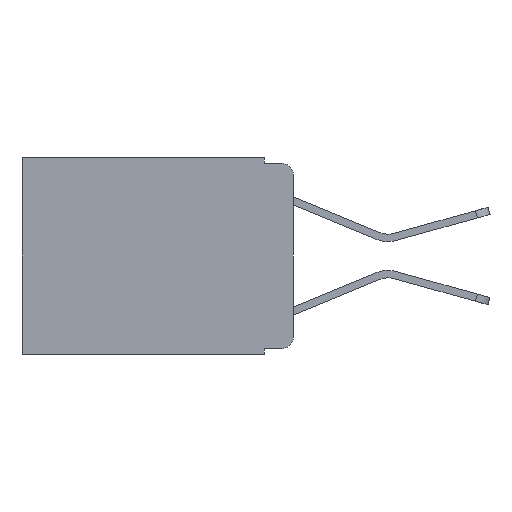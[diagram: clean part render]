
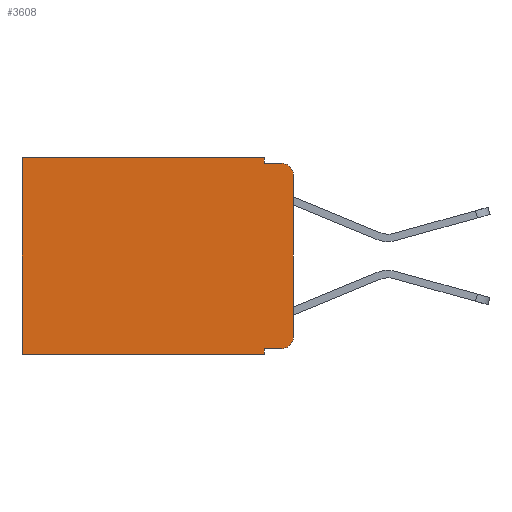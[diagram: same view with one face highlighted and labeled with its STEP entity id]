
A CAD part, left-side view. The second image highlights one B-rep face of the part: STEP entity #3608.
In plain terms, the highlighted planar face has unit normal (-1, 0, 0).
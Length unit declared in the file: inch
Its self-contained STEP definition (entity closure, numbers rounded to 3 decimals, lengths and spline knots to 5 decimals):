
#330 = VERTEX_POINT ( 'NONE', #3172 ) ;
#378 = ORIENTED_EDGE ( 'NONE', *, *, #8290, .F. ) ;
#444 = DIRECTION ( 'NONE',  ( 0., 0., -1. ) ) ;
#503 = CARTESIAN_POINT ( 'NONE',  ( 0.298, 0.051, -0.343 ) ) ;
#592 = CARTESIAN_POINT ( 'NONE',  ( 0.298, 0.02, -0.333 ) ) ;
#918 = CARTESIAN_POINT ( 'NONE',  ( 0.298, 0.051, 0. ) ) ;
#926 = VERTEX_POINT ( 'NONE', #20212 ) ;
#1026 = EDGE_CURVE ( 'NONE', #15799, #330, #22516, .T. ) ;
#1278 = LINE ( 'NONE', #4128, #19422 ) ;
#1350 = AXIS2_PLACEMENT_3D ( 'NONE', #12746, #19633, #444 ) ;
#1953 = VERTEX_POINT ( 'NONE', #12232 ) ;
#1965 = EDGE_CURVE ( 'NONE', #20426, #7676, #14026, .T. ) ;
#2195 = VECTOR ( 'NONE', #8801, 39.37008 ) ;
#2557 = VERTEX_POINT ( 'NONE', #918 ) ;
#2786 = LINE ( 'NONE', #15776, #2195 ) ;
#3076 = DIRECTION ( 'NONE',  ( 0., 0., -1. ) ) ;
#3172 = CARTESIAN_POINT ( 'NONE',  ( 0.298, 0.02, -0.01 ) ) ;
#3275 = VERTEX_POINT ( 'NONE', #503 ) ;
#3299 = ORIENTED_EDGE ( 'NONE', *, *, #6806, .T. ) ;
#3582 = DIRECTION ( 'NONE',  ( 0., 1., 0. ) ) ;
#3608 = ADVANCED_FACE ( 'NONE', ( #9942 ), #6311, .F. ) ;
#3767 = LINE ( 'NONE', #5191, #7946 ) ;
#4128 = CARTESIAN_POINT ( 'NONE',  ( 0.298, 0., 0. ) ) ;
#4423 = EDGE_CURVE ( 'NONE', #20426, #3275, #3767, .T. ) ;
#4692 = CARTESIAN_POINT ( 'NONE',  ( 0.298, 0., -0.343 ) ) ;
#5191 = CARTESIAN_POINT ( 'NONE',  ( 0.298, 0.051, 0. ) ) ;
#5262 = DIRECTION ( 'NONE',  ( -1., 0., 0. ) ) ;
#5292 = ORIENTED_EDGE ( 'NONE', *, *, #16869, .F. ) ;
#5762 = CARTESIAN_POINT ( 'NONE',  ( 0.298, 0.051, -0.333 ) ) ;
#5862 = ORIENTED_EDGE ( 'NONE', *, *, #11166, .T. ) ;
#5957 = DIRECTION ( 'NONE',  ( 0., 0., -1. ) ) ;
#6195 = VECTOR ( 'NONE', #11718, 39.37008 ) ;
#6311 = PLANE ( 'NONE',  #1350 ) ;
#6524 = DIRECTION ( 'NONE',  ( 0., 0., -1. ) ) ;
#6772 = LINE ( 'NONE', #22443, #20555 ) ;
#6806 = EDGE_CURVE ( 'NONE', #7155, #926, #21037, .T. ) ;
#7155 = VERTEX_POINT ( 'NONE', #19468 ) ;
#7283 = VECTOR ( 'NONE', #22437, 39.37008 ) ;
#7502 = ORIENTED_EDGE ( 'NONE', *, *, #1026, .T. ) ;
#7676 = VERTEX_POINT ( 'NONE', #592 ) ;
#7946 = VECTOR ( 'NONE', #6524, 39.37008 ) ;
#8290 = EDGE_CURVE ( 'NONE', #15799, #1953, #1278, .T. ) ;
#8801 = DIRECTION ( 'NONE',  ( 0., 0., -1. ) ) ;
#9430 = VECTOR ( 'NONE', #16887, 39.37008 ) ;
#9852 = VERTEX_POINT ( 'NONE', #20688 ) ;
#9942 = FACE_OUTER_BOUND ( 'NONE', #10870, .T. ) ;
#10552 = ORIENTED_EDGE ( 'NONE', *, *, #4423, .F. ) ;
#10700 = AXIS2_PLACEMENT_3D ( 'NONE', #15721, #5262, #17434 ) ;
#10870 = EDGE_LOOP ( 'NONE', ( #378, #7502, #17818, #5292, #5862, #3299, #17269, #10552, #11100, #19688 ) ) ;
#11100 = ORIENTED_EDGE ( 'NONE', *, *, #1965, .T. ) ;
#11166 = EDGE_CURVE ( 'NONE', #2557, #7155, #17694, .T. ) ;
#11718 = DIRECTION ( 'NONE',  ( 0., 1., 0. ) ) ;
#11940 = LINE ( 'NONE', #4692, #6195 ) ;
#12232 = CARTESIAN_POINT ( 'NONE',  ( 0.298, 0., -0.313 ) ) ;
#12289 = DIRECTION ( 'NONE',  ( 0., -1., 0. ) ) ;
#12746 = CARTESIAN_POINT ( 'NONE',  ( 0.298, 0., 0. ) ) ;
#13658 = DIRECTION ( 'NONE',  ( -1., 0., 0. ) ) ;
#14026 = LINE ( 'NONE', #19679, #9430 ) ;
#14209 = CARTESIAN_POINT ( 'NONE',  ( 0.298, 0., 0. ) ) ;
#15721 = CARTESIAN_POINT ( 'NONE',  ( 0.298, 0.02, -0.313 ) ) ;
#15776 = CARTESIAN_POINT ( 'NONE',  ( 0.298, 0.051, 0. ) ) ;
#15799 = VERTEX_POINT ( 'NONE', #22326 ) ;
#16662 = EDGE_CURVE ( 'NONE', #3275, #926, #11940, .T. ) ;
#16869 = EDGE_CURVE ( 'NONE', #2557, #9852, #2786, .T. ) ;
#16887 = DIRECTION ( 'NONE',  ( 0., -1., 0. ) ) ;
#17269 = ORIENTED_EDGE ( 'NONE', *, *, #16662, .F. ) ;
#17434 = DIRECTION ( 'NONE',  ( 0., 0., -1. ) ) ;
#17694 = LINE ( 'NONE', #14209, #18224 ) ;
#17818 = ORIENTED_EDGE ( 'NONE', *, *, #22482, .F. ) ;
#18224 = VECTOR ( 'NONE', #3582, 39.37008 ) ;
#18571 = CARTESIAN_POINT ( 'NONE',  ( 0.298, 0.02, -0.03 ) ) ;
#18747 = CIRCLE ( 'NONE', #10700, 0.02 ) ;
#19422 = VECTOR ( 'NONE', #5957, 39.37008 ) ;
#19468 = CARTESIAN_POINT ( 'NONE',  ( 0.298, 0.473, 0. ) ) ;
#19633 = DIRECTION ( 'NONE',  ( 1., 0., 0. ) ) ;
#19679 = CARTESIAN_POINT ( 'NONE',  ( 0.298, 0.051, -0.333 ) ) ;
#19688 = ORIENTED_EDGE ( 'NONE', *, *, #20872, .T. ) ;
#20212 = CARTESIAN_POINT ( 'NONE',  ( 0.298, 0.473, -0.343 ) ) ;
#20426 = VERTEX_POINT ( 'NONE', #5762 ) ;
#20529 = AXIS2_PLACEMENT_3D ( 'NONE', #18571, #13658, #3076 ) ;
#20555 = VECTOR ( 'NONE', #12289, 39.37008 ) ;
#20688 = CARTESIAN_POINT ( 'NONE',  ( 0.298, 0.051, -0.01 ) ) ;
#20872 = EDGE_CURVE ( 'NONE', #7676, #1953, #18747, .T. ) ;
#21037 = LINE ( 'NONE', #21796, #7283 ) ;
#21796 = CARTESIAN_POINT ( 'NONE',  ( 0.298, 0.473, 0. ) ) ;
#22326 = CARTESIAN_POINT ( 'NONE',  ( 0.298, 0., -0.03 ) ) ;
#22437 = DIRECTION ( 'NONE',  ( 0., 0., -1. ) ) ;
#22443 = CARTESIAN_POINT ( 'NONE',  ( 0.298, 0.051, -0.01 ) ) ;
#22482 = EDGE_CURVE ( 'NONE', #9852, #330, #6772, .T. ) ;
#22516 = CIRCLE ( 'NONE', #20529, 0.02 ) ;
